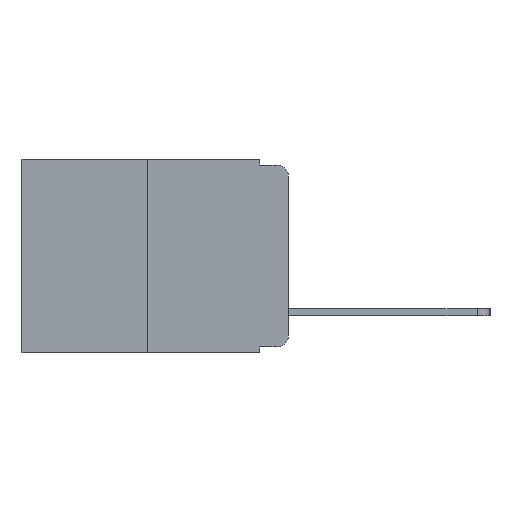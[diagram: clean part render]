
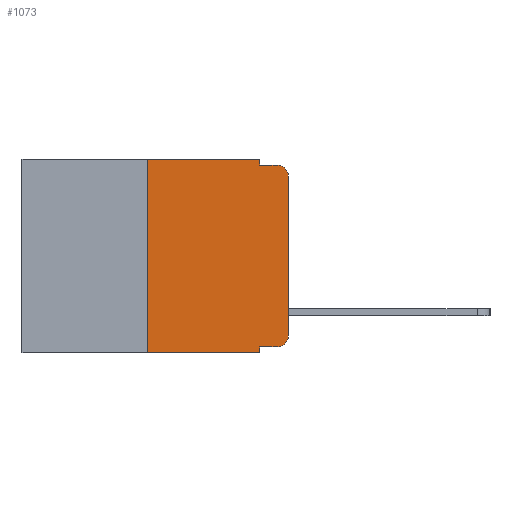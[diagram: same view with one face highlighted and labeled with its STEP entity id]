
A CAD part, left-side view. The second image highlights one B-rep face of the part: STEP entity #1073.
In plain terms, the highlighted planar face has unit normal (-1, 0, 0).
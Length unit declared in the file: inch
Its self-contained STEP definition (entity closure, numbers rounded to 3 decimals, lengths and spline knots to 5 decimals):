
#3 = ORIENTED_EDGE ( 'NONE', *, *, #6564, .F. ) ;
#43 = ORIENTED_EDGE ( 'NONE', *, *, #18737, .F. ) ;
#181 = EDGE_LOOP ( 'NONE', ( #1594, #8244, #8215, #3, #43, #12658, #18900, #18343, #417, #6939 ) ) ;
#364 = LINE ( 'NONE', #14830, #17002 ) ;
#417 = ORIENTED_EDGE ( 'NONE', *, *, #978, .T. ) ;
#479 = DIRECTION ( 'NONE',  ( -1., 0., 0. ) ) ;
#842 = CARTESIAN_POINT ( 'NONE',  ( 0., 0.473, 0. ) ) ;
#978 = EDGE_CURVE ( 'NONE', #6328, #2324, #364, .T. ) ;
#1073 = ADVANCED_FACE ( 'NONE', ( #19682 ), #6069, .F. ) ;
#1358 = LINE ( 'NONE', #4955, #13772 ) ;
#1594 = ORIENTED_EDGE ( 'NONE', *, *, #11897, .T. ) ;
#1689 = DIRECTION ( 'NONE',  ( 0., 0., -1. ) ) ;
#1936 = VECTOR ( 'NONE', #10018, 39.37008 ) ;
#2026 = VERTEX_POINT ( 'NONE', #20008 ) ;
#2103 = EDGE_CURVE ( 'NONE', #6328, #18306, #18466, .T. ) ;
#2309 = VECTOR ( 'NONE', #7847, 39.37008 ) ;
#2324 = VERTEX_POINT ( 'NONE', #3869 ) ;
#2984 = VERTEX_POINT ( 'NONE', #4173 ) ;
#3605 = LINE ( 'NONE', #17468, #4106 ) ;
#3869 = CARTESIAN_POINT ( 'NONE',  ( 0., 0.02, -0.333 ) ) ;
#3976 = VECTOR ( 'NONE', #12236, 39.37008 ) ;
#4106 = VECTOR ( 'NONE', #6434, 39.37008 ) ;
#4173 = CARTESIAN_POINT ( 'NONE',  ( 0., 0., -0.03 ) ) ;
#4314 = EDGE_CURVE ( 'NONE', #4673, #19338, #1358, .T. ) ;
#4673 = VERTEX_POINT ( 'NONE', #6534 ) ;
#4939 = CARTESIAN_POINT ( 'NONE',  ( 0., 0.473, 0. ) ) ;
#4955 = CARTESIAN_POINT ( 'NONE',  ( 0., 0.25, 0. ) ) ;
#5447 = DIRECTION ( 'NONE',  ( 0., -1., 0. ) ) ;
#5724 = EDGE_CURVE ( 'NONE', #4673, #18306, #17860, .T. ) ;
#6069 = PLANE ( 'NONE',  #17512 ) ;
#6328 = VERTEX_POINT ( 'NONE', #10449 ) ;
#6424 = VECTOR ( 'NONE', #7738, 39.37008 ) ;
#6434 = DIRECTION ( 'NONE',  ( 0., 0., 1. ) ) ;
#6435 = DIRECTION ( 'NONE',  ( 0., 0., 1. ) ) ;
#6534 = CARTESIAN_POINT ( 'NONE',  ( 0., 0.25, -0.343 ) ) ;
#6564 = EDGE_CURVE ( 'NONE', #2026, #16168, #10977, .T. ) ;
#6737 = DIRECTION ( 'NONE',  ( 0., -1., 0. ) ) ;
#6939 = ORIENTED_EDGE ( 'NONE', *, *, #19625, .T. ) ;
#6961 = CARTESIAN_POINT ( 'NONE',  ( 0., 0.473, -0.343 ) ) ;
#7626 = EDGE_CURVE ( 'NONE', #16168, #15743, #18525, .T. ) ;
#7738 = DIRECTION ( 'NONE',  ( 0., -1., 0. ) ) ;
#7847 = DIRECTION ( 'NONE',  ( 0., 0., -1. ) ) ;
#8215 = ORIENTED_EDGE ( 'NONE', *, *, #7626, .F. ) ;
#8244 = ORIENTED_EDGE ( 'NONE', *, *, #10849, .T. ) ;
#8317 = LINE ( 'NONE', #842, #3976 ) ;
#8763 = CIRCLE ( 'NONE', #17364, 0.02 ) ;
#8849 = CARTESIAN_POINT ( 'NONE',  ( 0., 0.25, 0. ) ) ;
#8972 = VECTOR ( 'NONE', #6737, 39.37008 ) ;
#9776 = CARTESIAN_POINT ( 'NONE',  ( 0., 0.051, 0. ) ) ;
#10018 = DIRECTION ( 'NONE',  ( 0., 0., -1. ) ) ;
#10290 = CARTESIAN_POINT ( 'NONE',  ( 0., 0.02, -0.03 ) ) ;
#10415 = DIRECTION ( 'NONE',  ( 0., 0., -1. ) ) ;
#10449 = CARTESIAN_POINT ( 'NONE',  ( 0., 0.051, -0.333 ) ) ;
#10737 = CARTESIAN_POINT ( 'NONE',  ( 0., 0.02, -0.01 ) ) ;
#10849 = EDGE_CURVE ( 'NONE', #2984, #15743, #16172, .T. ) ;
#10977 = LINE ( 'NONE', #18884, #2309 ) ;
#11443 = DIRECTION ( 'NONE',  ( -1., 0., 0. ) ) ;
#11652 = DIRECTION ( 'NONE',  ( 1., 0., 0. ) ) ;
#11897 = EDGE_CURVE ( 'NONE', #20038, #2984, #3605, .T. ) ;
#11900 = DIRECTION ( 'NONE',  ( 0., 0., -1. ) ) ;
#12236 = DIRECTION ( 'NONE',  ( 0., -1., 0. ) ) ;
#12444 = CARTESIAN_POINT ( 'NONE',  ( 0., 0., -0.313 ) ) ;
#12658 = ORIENTED_EDGE ( 'NONE', *, *, #4314, .F. ) ;
#13555 = CARTESIAN_POINT ( 'NONE',  ( 0., 0.051, -0.01 ) ) ;
#13772 = VECTOR ( 'NONE', #6435, 39.37008 ) ;
#14830 = CARTESIAN_POINT ( 'NONE',  ( 0., 0.051, -0.333 ) ) ;
#15103 = CARTESIAN_POINT ( 'NONE',  ( 0., 0.051, -0.343 ) ) ;
#15743 = VERTEX_POINT ( 'NONE', #10737 ) ;
#16168 = VERTEX_POINT ( 'NONE', #13555 ) ;
#16172 = CIRCLE ( 'NONE', #18297, 0.02 ) ;
#17002 = VECTOR ( 'NONE', #5447, 39.37008 ) ;
#17193 = CARTESIAN_POINT ( 'NONE',  ( 0., 0.051, -0.01 ) ) ;
#17364 = AXIS2_PLACEMENT_3D ( 'NONE', #20766, #11443, #1689 ) ;
#17468 = CARTESIAN_POINT ( 'NONE',  ( 0., 0., 0. ) ) ;
#17512 = AXIS2_PLACEMENT_3D ( 'NONE', #4939, #11652, #10415 ) ;
#17860 = LINE ( 'NONE', #6961, #8972 ) ;
#18297 = AXIS2_PLACEMENT_3D ( 'NONE', #10290, #479, #11900 ) ;
#18306 = VERTEX_POINT ( 'NONE', #15103 ) ;
#18343 = ORIENTED_EDGE ( 'NONE', *, *, #2103, .F. ) ;
#18466 = LINE ( 'NONE', #9776, #1936 ) ;
#18525 = LINE ( 'NONE', #17193, #6424 ) ;
#18737 = EDGE_CURVE ( 'NONE', #19338, #2026, #8317, .T. ) ;
#18884 = CARTESIAN_POINT ( 'NONE',  ( 0., 0.051, 0. ) ) ;
#18900 = ORIENTED_EDGE ( 'NONE', *, *, #5724, .T. ) ;
#19338 = VERTEX_POINT ( 'NONE', #8849 ) ;
#19625 = EDGE_CURVE ( 'NONE', #2324, #20038, #8763, .T. ) ;
#19682 = FACE_OUTER_BOUND ( 'NONE', #181, .T. ) ;
#20008 = CARTESIAN_POINT ( 'NONE',  ( 0., 0.051, 0. ) ) ;
#20038 = VERTEX_POINT ( 'NONE', #12444 ) ;
#20766 = CARTESIAN_POINT ( 'NONE',  ( 0., 0.02, -0.313 ) ) ;
